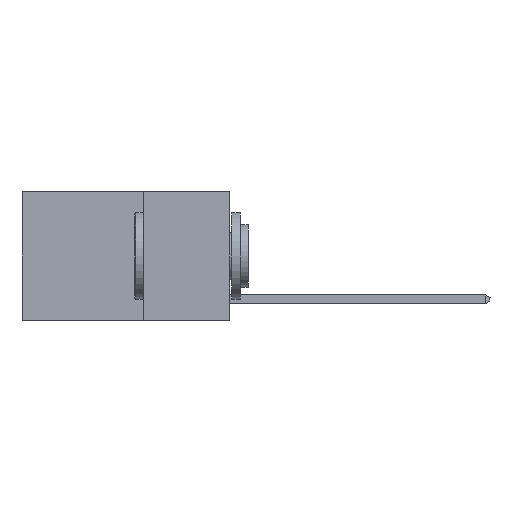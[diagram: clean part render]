
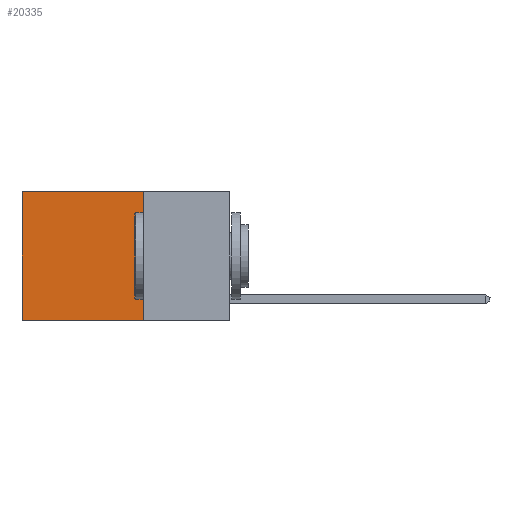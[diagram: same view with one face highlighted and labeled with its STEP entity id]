
A CAD part, left-side view. The second image highlights one B-rep face of the part: STEP entity #20335.
In plain terms, the highlighted planar face has unit normal (-1, 0, 0).
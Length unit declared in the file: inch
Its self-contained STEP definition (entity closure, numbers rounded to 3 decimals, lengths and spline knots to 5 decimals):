
#1843 = PLANE ( 'NONE',  #14281 ) ;
#2988 = ORIENTED_EDGE ( 'NONE', *, *, #25859, .T. ) ;
#3995 = VECTOR ( 'NONE', #23657, 39.37008 ) ;
#4280 = CARTESIAN_POINT ( 'NONE',  ( 0.2625, 0.25, -0.37 ) ) ;
#5904 = DIRECTION ( 'NONE',  ( 0., 0., -1. ) ) ;
#6653 = LINE ( 'NONE', #24437, #7932 ) ;
#6824 = LINE ( 'NONE', #9417, #26287 ) ;
#7049 = ORIENTED_EDGE ( 'NONE', *, *, #8363, .F. ) ;
#7932 = VECTOR ( 'NONE', #13427, 39.37008 ) ;
#8190 = LINE ( 'NONE', #19607, #3995 ) ;
#8363 = EDGE_CURVE ( 'NONE', #23394, #9057, #20125, .T. ) ;
#8679 = EDGE_LOOP ( 'NONE', ( #12099, #21678, #7049, #2988 ) ) ;
#9056 = CARTESIAN_POINT ( 'NONE',  ( 0.2625, 0.6, 0. ) ) ;
#9057 = VERTEX_POINT ( 'NONE', #4280 ) ;
#9417 = CARTESIAN_POINT ( 'NONE',  ( 0.2625, 0.6, 0. ) ) ;
#12099 = ORIENTED_EDGE ( 'NONE', *, *, #12502, .T. ) ;
#12502 = EDGE_CURVE ( 'NONE', #21804, #25052, #6824, .T. ) ;
#13427 = DIRECTION ( 'NONE',  ( 0., 1., 0. ) ) ;
#14281 = AXIS2_PLACEMENT_3D ( 'NONE', #19466, #14727, #5904 ) ;
#14727 = DIRECTION ( 'NONE',  ( 1., 0., 0. ) ) ;
#14770 = EDGE_CURVE ( 'NONE', #9057, #25052, #8190, .T. ) ;
#14874 = FACE_OUTER_BOUND ( 'NONE', #8679, .T. ) ;
#15855 = VECTOR ( 'NONE', #17828, 39.37008 ) ;
#17727 = CARTESIAN_POINT ( 'NONE',  ( 0.2625, 0.6, -0.37 ) ) ;
#17828 = DIRECTION ( 'NONE',  ( 0., 0., -1. ) ) ;
#19466 = CARTESIAN_POINT ( 'NONE',  ( 0.2625, 0.25, 0. ) ) ;
#19607 = CARTESIAN_POINT ( 'NONE',  ( 0.2625, 0.25, -0.37 ) ) ;
#20125 = LINE ( 'NONE', #24634, #15855 ) ;
#20335 = ADVANCED_FACE ( 'NONE', ( #14874 ), #1843, .F. ) ;
#20686 = DIRECTION ( 'NONE',  ( 0., 0., -1. ) ) ;
#21179 = CARTESIAN_POINT ( 'NONE',  ( 0.2625, 0.25, 0. ) ) ;
#21678 = ORIENTED_EDGE ( 'NONE', *, *, #14770, .F. ) ;
#21804 = VERTEX_POINT ( 'NONE', #9056 ) ;
#23394 = VERTEX_POINT ( 'NONE', #21179 ) ;
#23657 = DIRECTION ( 'NONE',  ( 0., 1., 0. ) ) ;
#24437 = CARTESIAN_POINT ( 'NONE',  ( 0.2625, 0.25, 0. ) ) ;
#24634 = CARTESIAN_POINT ( 'NONE',  ( 0.2625, 0.25, 0. ) ) ;
#25052 = VERTEX_POINT ( 'NONE', #17727 ) ;
#25859 = EDGE_CURVE ( 'NONE', #23394, #21804, #6653, .T. ) ;
#26287 = VECTOR ( 'NONE', #20686, 39.37008 ) ;
